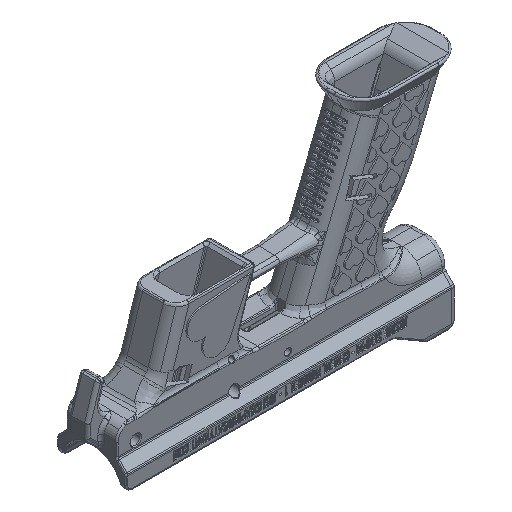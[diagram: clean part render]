
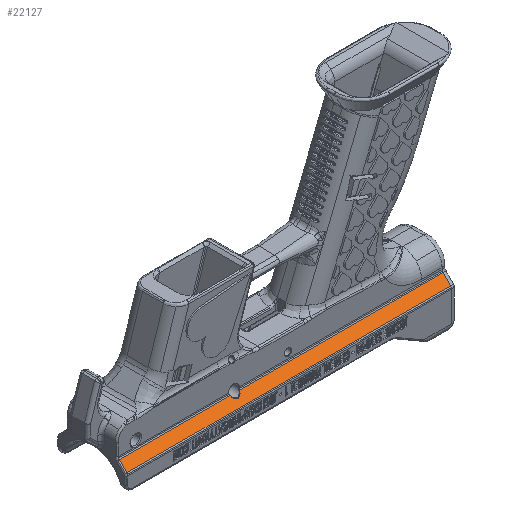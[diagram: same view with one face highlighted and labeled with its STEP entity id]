
A CAD part, isometric view. The second image highlights one B-rep face of the part: STEP entity #22127.
In plain terms, the highlighted planar face has unit normal (0, -0.707, 0.707).
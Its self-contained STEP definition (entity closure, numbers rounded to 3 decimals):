
#1621 = B_SPLINE_CURVE_WITH_KNOTS ( 'NONE', 3,
 ( #36339, #82451, #48992, #139741, #81706, #127109, #25186 ),
 .UNSPECIFIED., .F., .F.,
 ( 4, 1, 1, 1, 4 ),
 ( -1.109, -0.475, 0.158, 0.475, 1.109 ),
 .UNSPECIFIED. ) ;
#2847 = EDGE_CURVE ( 'NONE', #70120, #73030, #46355, .T. ) ;
#3976 = ORIENTED_EDGE ( 'NONE', *, *, #75370, .F. ) ;
#8293 = CARTESIAN_POINT ( 'NONE',  ( -2.415, -16.586, -81.586 ) ) ;
#9753 = CARTESIAN_POINT ( 'NONE',  ( -2.434, -16.625, -81.625 ) ) ;
#11227 = EDGE_CURVE ( 'NONE', #73030, #40657, #128641, .T. ) ;
#12844 = DIRECTION ( 'NONE',  ( 0., 0.707, 0.707 ) ) ;
#15891 = VECTOR ( 'NONE', #48339, 1000. ) ;
#20594 = LINE ( 'NONE', #112856, #92072 ) ;
#20898 = CARTESIAN_POINT ( 'NONE',  ( -2.444, -16.644, -81.644 ) ) ;
#22127 = ADVANCED_FACE ( 'NONE', ( #90794 ), #55138, .T. ) ;
#22346 = CARTESIAN_POINT ( 'NONE',  ( -8.566, -16.625, -81.625 ) ) ;
#23088 = CARTESIAN_POINT ( 'NONE',  ( -26.657, -19., -84. ) ) ;
#24714 = VECTOR ( 'NONE', #12844, 1000. ) ;
#25186 = CARTESIAN_POINT ( 'NONE',  ( -2.444, -16.644, -81.644 ) ) ;
#28210 = CARTESIAN_POINT ( 'NONE',  ( 126.981, -16.586, -81.586 ) ) ;
#29396 = CARTESIAN_POINT ( 'NONE',  ( -79., -21.414, -86.414 ) ) ;
#33153 = CARTESIAN_POINT ( 'NONE',  ( -8.585, -16.586, -81.586 ) ) ;
#33911 = B_SPLINE_CURVE_WITH_KNOTS ( 'NONE', 3,
 ( #102697, #93740, #22346, #70679 ),
 .UNSPECIFIED., .F., .F.,
 ( 4, 4 ),
 ( -0.79, -0.781 ),
 .UNSPECIFIED. ) ;
#36339 = CARTESIAN_POINT ( 'NONE',  ( -8.556, -16.644, -81.644 ) ) ;
#40026 = VECTOR ( 'NONE', #127057, 1000. ) ;
#40657 = VERTEX_POINT ( 'NONE', #33153 ) ;
#41924 = CARTESIAN_POINT ( 'NONE',  ( -2.444, -16.644, -81.644 ) ) ;
#44836 = VERTEX_POINT ( 'NONE', #143276 ) ;
#45154 = CARTESIAN_POINT ( 'NONE',  ( -2.415, -16.586, -81.586 ) ) ;
#46355 = LINE ( 'NONE', #80554, #24714 ) ;
#46580 = EDGE_LOOP ( 'NONE', ( #137460, #3976, #105633, #80938, #60850, #124355, #120270, #143076 ) ) ;
#48203 = LINE ( 'NONE', #81661, #40026 ) ;
#48339 = DIRECTION ( 'NONE',  ( 1., 0., 0. ) ) ;
#48992 = CARTESIAN_POINT ( 'NONE',  ( -7.218, -18.331, -83.331 ) ) ;
#53330 = VERTEX_POINT ( 'NONE', #84029 ) ;
#53843 = LINE ( 'NONE', #54580, #88144 ) ;
#54580 = CARTESIAN_POINT ( 'NONE',  ( 0.014, -16.586, -81.586 ) ) ;
#54906 = VERTEX_POINT ( 'NONE', #45154 ) ;
#55138 = PLANE ( 'NONE',  #74853 ) ;
#60850 = ORIENTED_EDGE ( 'NONE', *, *, #90514, .F. ) ;
#68478 = DIRECTION ( 'NONE',  ( 0., -0.707, 0.707 ) ) ;
#69916 = EDGE_CURVE ( 'NONE', #105121, #53330, #20594, .T. ) ;
#70120 = VERTEX_POINT ( 'NONE', #29396 ) ;
#70679 = CARTESIAN_POINT ( 'NONE',  ( -8.556, -16.644, -81.644 ) ) ;
#72107 = CARTESIAN_POINT ( 'NONE',  ( 0.014, -16.586, -81.586 ) ) ;
#73030 = VERTEX_POINT ( 'NONE', #108360 ) ;
#73789 = VERTEX_POINT ( 'NONE', #41924 ) ;
#74853 = AXIS2_PLACEMENT_3D ( 'NONE', #23088, #68478, #113870 ) ;
#75370 = EDGE_CURVE ( 'NONE', #53330, #70120, #48203, .T. ) ;
#77406 = B_SPLINE_CURVE_WITH_KNOTS ( 'NONE', 3,
 ( #20898, #9753, #110196, #8293 ),
 .UNSPECIFIED., .F., .F.,
 ( 4, 4 ),
 ( -0.468, -0.459 ),
 .UNSPECIFIED. ) ;
#80554 = CARTESIAN_POINT ( 'NONE',  ( -79., -17.5, -82.5 ) ) ;
#80938 = ORIENTED_EDGE ( 'NONE', *, *, #99207, .F. ) ;
#81661 = CARTESIAN_POINT ( 'NONE',  ( -0.583, -21.414, -86.414 ) ) ;
#81706 = CARTESIAN_POINT ( 'NONE',  ( -3.527, -18.057, -83.057 ) ) ;
#82451 = CARTESIAN_POINT ( 'NONE',  ( -8.246, -17.268, -82.268 ) ) ;
#84029 = CARTESIAN_POINT ( 'NONE',  ( 126.981, -21.414, -86.414 ) ) ;
#88144 = VECTOR ( 'NONE', #121512, 1000. ) ;
#90514 = EDGE_CURVE ( 'NONE', #73789, #54906, #77406, .T. ) ;
#90794 = FACE_OUTER_BOUND ( 'NONE', #46580, .T. ) ;
#92072 = VECTOR ( 'NONE', #144880, 1000. ) ;
#93740 = CARTESIAN_POINT ( 'NONE',  ( -8.576, -16.606, -81.606 ) ) ;
#99207 = EDGE_CURVE ( 'NONE', #54906, #105121, #53843, .T. ) ;
#99742 = EDGE_CURVE ( 'NONE', #40657, #44836, #33911, .T. ) ;
#102697 = CARTESIAN_POINT ( 'NONE',  ( -8.585, -16.586, -81.586 ) ) ;
#105121 = VERTEX_POINT ( 'NONE', #28210 ) ;
#105633 = ORIENTED_EDGE ( 'NONE', *, *, #69916, .F. ) ;
#108360 = CARTESIAN_POINT ( 'NONE',  ( -79., -16.586, -81.586 ) ) ;
#110196 = CARTESIAN_POINT ( 'NONE',  ( -2.424, -16.606, -81.606 ) ) ;
#112856 = CARTESIAN_POINT ( 'NONE',  ( 126.981, -10., -75. ) ) ;
#113870 = DIRECTION ( 'NONE',  ( -1., 0., 0. ) ) ;
#120270 = ORIENTED_EDGE ( 'NONE', *, *, #99742, .F. ) ;
#121512 = DIRECTION ( 'NONE',  ( 1., 0., 0. ) ) ;
#124355 = ORIENTED_EDGE ( 'NONE', *, *, #128629, .F. ) ;
#127057 = DIRECTION ( 'NONE',  ( -1., 0., 0. ) ) ;
#127109 = CARTESIAN_POINT ( 'NONE',  ( -2.754, -17.268, -82.268 ) ) ;
#128629 = EDGE_CURVE ( 'NONE', #44836, #73789, #1621, .T. ) ;
#128641 = LINE ( 'NONE', #72107, #15891 ) ;
#137460 = ORIENTED_EDGE ( 'NONE', *, *, #2847, .F. ) ;
#139741 = CARTESIAN_POINT ( 'NONE',  ( -5.29, -18.644, -83.644 ) ) ;
#143076 = ORIENTED_EDGE ( 'NONE', *, *, #11227, .F. ) ;
#143276 = CARTESIAN_POINT ( 'NONE',  ( -8.556, -16.644, -81.644 ) ) ;
#144880 = DIRECTION ( 'NONE',  ( 0., -0.707, -0.707 ) ) ;
